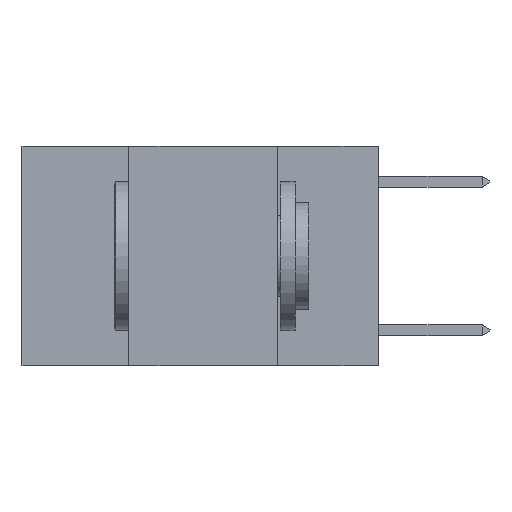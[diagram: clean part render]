
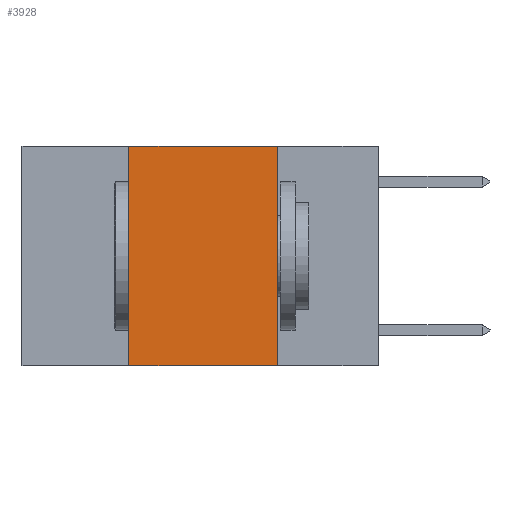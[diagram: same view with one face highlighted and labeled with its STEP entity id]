
A CAD part, left-side view. The second image highlights one B-rep face of the part: STEP entity #3928.
In plain terms, the highlighted planar face has unit normal (-1, 0, 0).
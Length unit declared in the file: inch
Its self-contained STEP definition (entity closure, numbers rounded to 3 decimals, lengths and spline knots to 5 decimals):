
#539 = CARTESIAN_POINT ( 'NONE',  ( 0., 0.17, -0.37 ) ) ;
#858 = VECTOR ( 'NONE', #2650, 39.37008 ) ;
#1117 = EDGE_LOOP ( 'NONE', ( #5043, #11248, #9146, #2269 ) ) ;
#1372 = VECTOR ( 'NONE', #2455, 39.37008 ) ;
#1428 = CARTESIAN_POINT ( 'NONE',  ( 0., 0.6, 0. ) ) ;
#1847 = FACE_OUTER_BOUND ( 'NONE', #1117, .T. ) ;
#1934 = VERTEX_POINT ( 'NONE', #539 ) ;
#2269 = ORIENTED_EDGE ( 'NONE', *, *, #5785, .T. ) ;
#2415 = DIRECTION ( 'NONE',  ( 0., 0., -1. ) ) ;
#2455 = DIRECTION ( 'NONE',  ( 0., 0., -1. ) ) ;
#2650 = DIRECTION ( 'NONE',  ( 0., 0., 1. ) ) ;
#2886 = CARTESIAN_POINT ( 'NONE',  ( 0., 0.42, -0.37 ) ) ;
#3183 = DIRECTION ( 'NONE',  ( 0., -1., 0. ) ) ;
#3485 = LINE ( 'NONE', #4495, #858 ) ;
#3676 = CARTESIAN_POINT ( 'NONE',  ( 0., 0.6, 0. ) ) ;
#3928 = ADVANCED_FACE ( 'NONE', ( #1847 ), #6146, .F. ) ;
#3973 = LINE ( 'NONE', #10825, #1372 ) ;
#4495 = CARTESIAN_POINT ( 'NONE',  ( 0., 0.42, 0. ) ) ;
#4777 = CARTESIAN_POINT ( 'NONE',  ( 0., 0.17, 0. ) ) ;
#5043 = ORIENTED_EDGE ( 'NONE', *, *, #10139, .F. ) ;
#5397 = EDGE_CURVE ( 'NONE', #8954, #10466, #3485, .T. ) ;
#5785 = EDGE_CURVE ( 'NONE', #8954, #1934, #8962, .T. ) ;
#5871 = CARTESIAN_POINT ( 'NONE',  ( 0., 0.42, 0. ) ) ;
#6146 = PLANE ( 'NONE',  #10161 ) ;
#7679 = EDGE_CURVE ( 'NONE', #10466, #7869, #9775, .T. ) ;
#7869 = VERTEX_POINT ( 'NONE', #4777 ) ;
#8045 = DIRECTION ( 'NONE',  ( 1., 0., 0. ) ) ;
#8741 = CARTESIAN_POINT ( 'NONE',  ( 0., 0.6, -0.37 ) ) ;
#8954 = VERTEX_POINT ( 'NONE', #2886 ) ;
#8962 = LINE ( 'NONE', #8741, #12044 ) ;
#9146 = ORIENTED_EDGE ( 'NONE', *, *, #5397, .F. ) ;
#9775 = LINE ( 'NONE', #3676, #11999 ) ;
#10139 = EDGE_CURVE ( 'NONE', #7869, #1934, #3973, .T. ) ;
#10161 = AXIS2_PLACEMENT_3D ( 'NONE', #1428, #8045, #2415 ) ;
#10466 = VERTEX_POINT ( 'NONE', #5871 ) ;
#10825 = CARTESIAN_POINT ( 'NONE',  ( 0., 0.17, 0. ) ) ;
#11248 = ORIENTED_EDGE ( 'NONE', *, *, #7679, .F. ) ;
#11999 = VECTOR ( 'NONE', #12022, 39.37008 ) ;
#12022 = DIRECTION ( 'NONE',  ( 0., -1., 0. ) ) ;
#12044 = VECTOR ( 'NONE', #3183, 39.37008 ) ;
